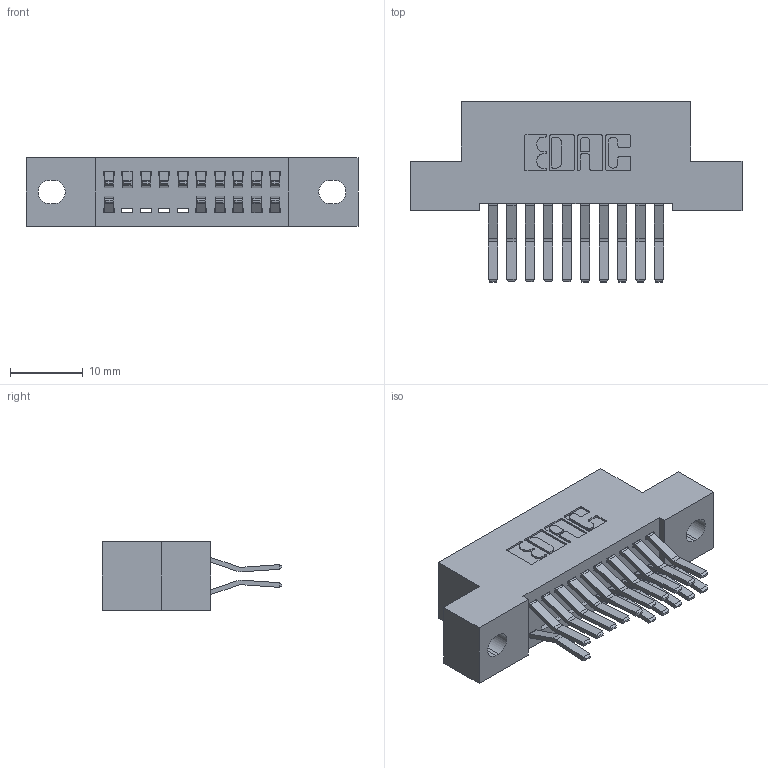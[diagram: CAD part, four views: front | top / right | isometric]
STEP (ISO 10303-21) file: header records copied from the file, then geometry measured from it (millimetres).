
FILE_DESCRIPTION (( 'STEP AP203' ), '1' );
FILE_NAME ('392-020-560-202.STEP', '2018-08-15T07:28:17', ( '' ), ( '' ), 'SwSTEP 2.0', 'SolidWorks 2016', '' );
FILE_SCHEMA (( 'CONFIG_CONTROL_DESIGN' ));
Length unit declared in the file: inch
Products named in the file (3): 342 Part_.128 Slot; 345-292-001_560 Tail; 392-020-560-202
Assembly tree (17 placements, depth 2):
  392-020-560-202
    342 Part_.128 Slot
    345-292-001_560 Tail  x16
Bounding box: 45.72 x 24.78 x 9.4 mm (x, y, z)
Volume: 3973.4 mm3; surface area: 5491.6 mm2
Topology: 17 solids, 17 shells, 1002 faces, 2971 edges, 1958 vertices
Faces by surface type: plane 670, cylinder 332
Entity records: 10535 total; most frequent: CARTESIAN_POINT 1802, ORIENTED_EDGE 1742, DIRECTION 1595, EDGE_CURVE 871, VECTOR 739, LINE 739, VERTEX_POINT 578, AXIS2_PLACEMENT_3D 428
